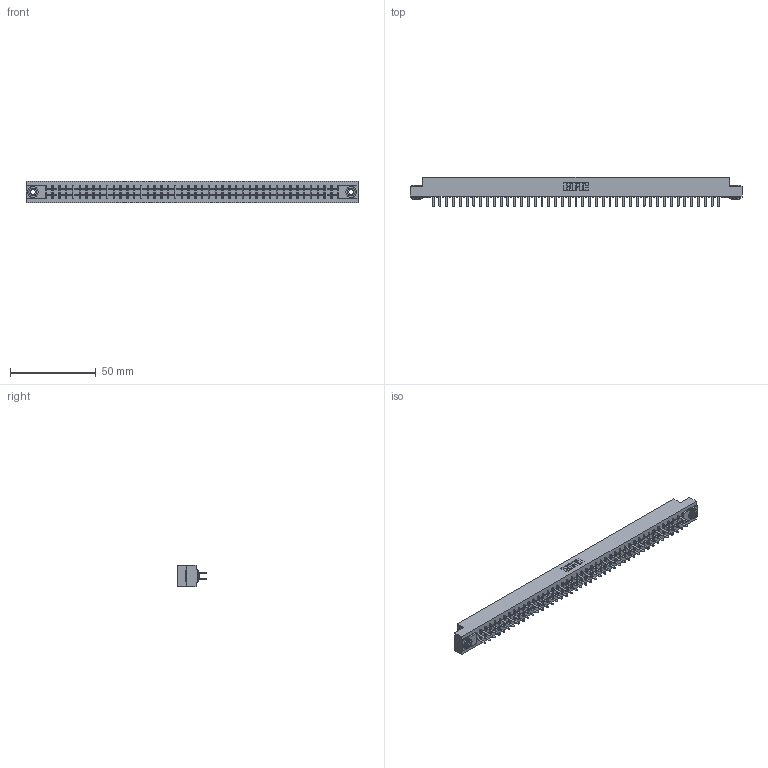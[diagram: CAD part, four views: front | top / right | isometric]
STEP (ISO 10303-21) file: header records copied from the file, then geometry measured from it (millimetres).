
FILE_DESCRIPTION (( 'STEP AP203' ), '1' );
FILE_NAME ('355-086-520-203.STEP', '2019-09-13T16:32:58', ( '' ), ( '' ), 'SwSTEP 2.0', 'SolidWorks 2016', '' );
FILE_SCHEMA (( 'CONFIG_CONTROL_DESIGN' ));
Length unit declared in the file: inch
Products named in the file (4): 305-290-001_520; 305 Part_.156 Dia; 355-086-520-203; 345-250-002_345-250-002-102
Assembly tree (89 placements, depth 2):
  355-086-520-203
    305 Part_.156 Dia
    305-290-001_520  x86
    345-250-002_345-250-002-102  x2
Bounding box: 193.4 x 17.09 x 12.7 mm (x, y, z)
Volume: 20168.9 mm3; surface area: 26013.3 mm2
Topology: 89 solids, 89 shells, 4124 faces, 11737 edges, 7590 vertices
Faces by surface type: plane 2414, cylinder 1530, sphere 172, cone 8
Entity records: 47381 total; most frequent: CARTESIAN_POINT 7820, ORIENTED_EDGE 7754, DIRECTION 7579, EDGE_CURVE 3877, VECTOR 3129, LINE 3129, VERTEX_POINT 2466, AXIS2_PLACEMENT_3D 2225
